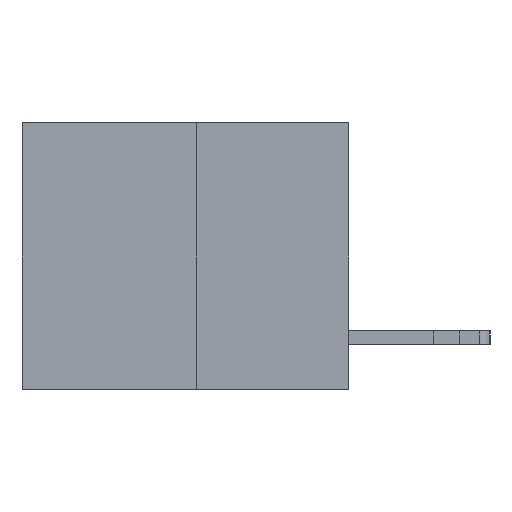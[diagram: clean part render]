
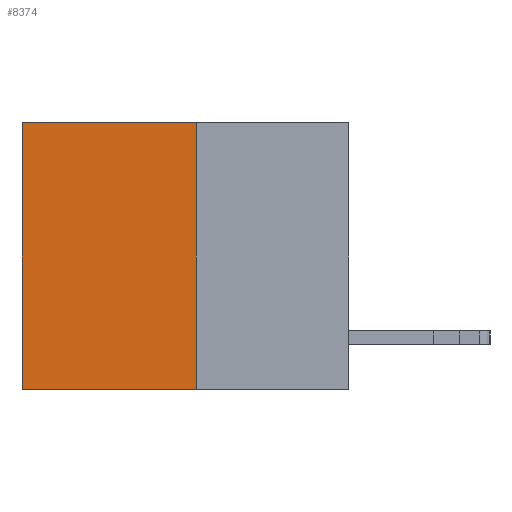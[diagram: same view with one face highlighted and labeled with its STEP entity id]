
A CAD part, left-side view. The second image highlights one B-rep face of the part: STEP entity #8374.
In plain terms, the highlighted planar face has unit normal (-1, 0, 0).
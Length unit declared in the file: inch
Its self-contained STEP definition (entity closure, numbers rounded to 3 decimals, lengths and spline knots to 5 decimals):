
#47 = DIRECTION ( 'NONE',  ( 1., 0., 0. ) ) ;
#275 = VERTEX_POINT ( 'NONE', #657 ) ;
#386 = ORIENTED_EDGE ( 'NONE', *, *, #14258, .T. ) ;
#657 = CARTESIAN_POINT ( 'NONE',  ( 0.3165, 0.6, -0.49 ) ) ;
#662 = DIRECTION ( 'NONE',  ( 0., 1., 0. ) ) ;
#1392 = ORIENTED_EDGE ( 'NONE', *, *, #16633, .F. ) ;
#2771 = CARTESIAN_POINT ( 'NONE',  ( 0.3165, 0.28, -0.49 ) ) ;
#2835 = LINE ( 'NONE', #16254, #17049 ) ;
#3807 = VERTEX_POINT ( 'NONE', #14750 ) ;
#4536 = EDGE_LOOP ( 'NONE', ( #386, #13589, #1392, #5052 ) ) ;
#4931 = VECTOR ( 'NONE', #15669, 39.37008 ) ;
#5052 = ORIENTED_EDGE ( 'NONE', *, *, #11865, .T. ) ;
#5269 = AXIS2_PLACEMENT_3D ( 'NONE', #2771, #47, #11448 ) ;
#8034 = LINE ( 'NONE', #11170, #4931 ) ;
#8374 = ADVANCED_FACE ( 'NONE', ( #12333 ), #9774, .F. ) ;
#9763 = CARTESIAN_POINT ( 'NONE',  ( 0.3165, 0.28, -0.49 ) ) ;
#9774 = PLANE ( 'NONE',  #5269 ) ;
#10842 = VERTEX_POINT ( 'NONE', #12674 ) ;
#11170 = CARTESIAN_POINT ( 'NONE',  ( 0.3165, 0.6, -0.49 ) ) ;
#11448 = DIRECTION ( 'NONE',  ( 0., 0., -1. ) ) ;
#11831 = DIRECTION ( 'NONE',  ( 0., 0., -1. ) ) ;
#11865 = EDGE_CURVE ( 'NONE', #14353, #3807, #15315, .T. ) ;
#12333 = FACE_OUTER_BOUND ( 'NONE', #4536, .T. ) ;
#12380 = VECTOR ( 'NONE', #18161, 39.37008 ) ;
#12674 = CARTESIAN_POINT ( 'NONE',  ( 0.3165, 0.28, -0.49 ) ) ;
#13302 = VECTOR ( 'NONE', #662, 39.37008 ) ;
#13589 = ORIENTED_EDGE ( 'NONE', *, *, #16104, .F. ) ;
#14258 = EDGE_CURVE ( 'NONE', #3807, #275, #8034, .T. ) ;
#14353 = VERTEX_POINT ( 'NONE', #17121 ) ;
#14750 = CARTESIAN_POINT ( 'NONE',  ( 0.3165, 0.6, 0. ) ) ;
#15315 = LINE ( 'NONE', #17481, #13302 ) ;
#15669 = DIRECTION ( 'NONE',  ( 0., 0., -1. ) ) ;
#16104 = EDGE_CURVE ( 'NONE', #10842, #275, #16203, .T. ) ;
#16203 = LINE ( 'NONE', #9763, #12380 ) ;
#16254 = CARTESIAN_POINT ( 'NONE',  ( 0.3165, 0.28, -0.49 ) ) ;
#16633 = EDGE_CURVE ( 'NONE', #14353, #10842, #2835, .T. ) ;
#17049 = VECTOR ( 'NONE', #11831, 39.37008 ) ;
#17121 = CARTESIAN_POINT ( 'NONE',  ( 0.3165, 0.28, 0. ) ) ;
#17481 = CARTESIAN_POINT ( 'NONE',  ( 0.3165, 0.28, 0. ) ) ;
#18161 = DIRECTION ( 'NONE',  ( 0., 1., 0. ) ) ;
